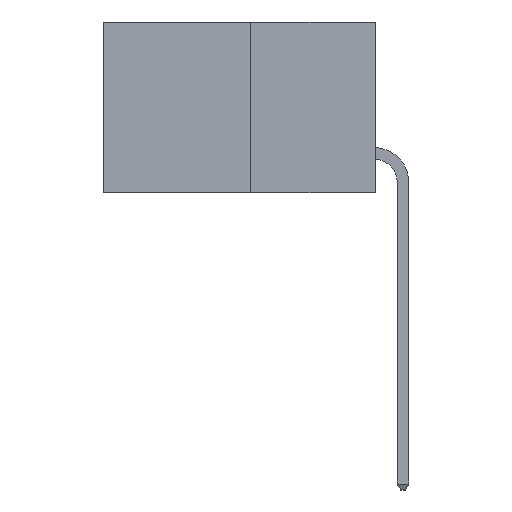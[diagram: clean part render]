
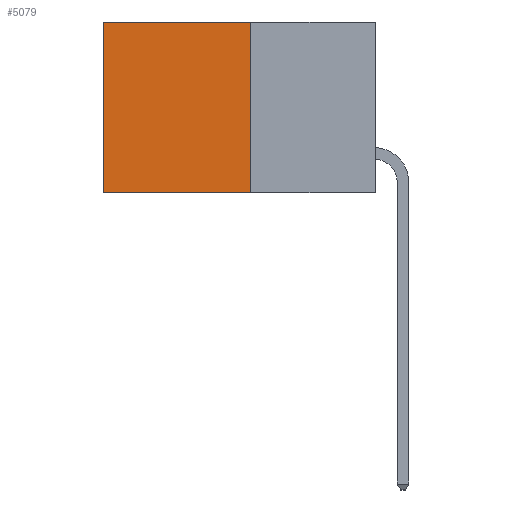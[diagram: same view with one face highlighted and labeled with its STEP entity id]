
A CAD part, left-side view. The second image highlights one B-rep face of the part: STEP entity #5079.
In plain terms, the highlighted planar face has unit normal (-1, 0, 0).
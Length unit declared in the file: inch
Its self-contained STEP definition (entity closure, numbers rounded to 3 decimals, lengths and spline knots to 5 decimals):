
#337 = CARTESIAN_POINT ( 'NONE',  ( 0.277, 0.27, -0.37 ) ) ;
#558 = VERTEX_POINT ( 'NONE', #2427 ) ;
#783 = VERTEX_POINT ( 'NONE', #798 ) ;
#798 = CARTESIAN_POINT ( 'NONE',  ( 0.277, 0.59, 0. ) ) ;
#1088 = VECTOR ( 'NONE', #7801, 39.37008 ) ;
#2061 = DIRECTION ( 'NONE',  ( 0., 1., 0. ) ) ;
#2107 = LINE ( 'NONE', #7609, #5890 ) ;
#2427 = CARTESIAN_POINT ( 'NONE',  ( 0.277, 0.27, 0. ) ) ;
#2670 = ORIENTED_EDGE ( 'NONE', *, *, #9119, .F. ) ;
#2933 = ORIENTED_EDGE ( 'NONE', *, *, #4155, .T. ) ;
#3074 = DIRECTION ( 'NONE',  ( 0., 0., -1. ) ) ;
#3082 = VECTOR ( 'NONE', #2061, 39.37008 ) ;
#3089 = VERTEX_POINT ( 'NONE', #337 ) ;
#3205 = AXIS2_PLACEMENT_3D ( 'NONE', #6696, #3332, #3304 ) ;
#3218 = ORIENTED_EDGE ( 'NONE', *, *, #8998, .T. ) ;
#3304 = DIRECTION ( 'NONE',  ( 0., 0., -1. ) ) ;
#3332 = DIRECTION ( 'NONE',  ( 1., 0., 0. ) ) ;
#3853 = VECTOR ( 'NONE', #3074, 39.37008 ) ;
#4155 = EDGE_CURVE ( 'NONE', #783, #6528, #5840, .T. ) ;
#4873 = LINE ( 'NONE', #5503, #3082 ) ;
#5079 = ADVANCED_FACE ( 'NONE', ( #6548 ), #5883, .F. ) ;
#5203 = LINE ( 'NONE', #7096, #1088 ) ;
#5503 = CARTESIAN_POINT ( 'NONE',  ( 0.277, 0.27, 0. ) ) ;
#5840 = LINE ( 'NONE', #7063, #3853 ) ;
#5883 = PLANE ( 'NONE',  #3205 ) ;
#5890 = VECTOR ( 'NONE', #7677, 39.37008 ) ;
#6528 = VERTEX_POINT ( 'NONE', #8076 ) ;
#6548 = FACE_OUTER_BOUND ( 'NONE', #8759, .T. ) ;
#6696 = CARTESIAN_POINT ( 'NONE',  ( 0.277, 0.27, -0.37 ) ) ;
#7063 = CARTESIAN_POINT ( 'NONE',  ( 0.277, 0.59, -0.37 ) ) ;
#7096 = CARTESIAN_POINT ( 'NONE',  ( 0.277, 0.27, -0.37 ) ) ;
#7609 = CARTESIAN_POINT ( 'NONE',  ( 0.277, 0.27, -0.37 ) ) ;
#7677 = DIRECTION ( 'NONE',  ( 0., 1., 0. ) ) ;
#7801 = DIRECTION ( 'NONE',  ( 0., 0., -1. ) ) ;
#8076 = CARTESIAN_POINT ( 'NONE',  ( 0.277, 0.59, -0.37 ) ) ;
#8607 = ORIENTED_EDGE ( 'NONE', *, *, #9608, .F. ) ;
#8759 = EDGE_LOOP ( 'NONE', ( #2933, #2670, #8607, #3218 ) ) ;
#8998 = EDGE_CURVE ( 'NONE', #558, #783, #4873, .T. ) ;
#9119 = EDGE_CURVE ( 'NONE', #3089, #6528, #2107, .T. ) ;
#9608 = EDGE_CURVE ( 'NONE', #558, #3089, #5203, .T. ) ;
